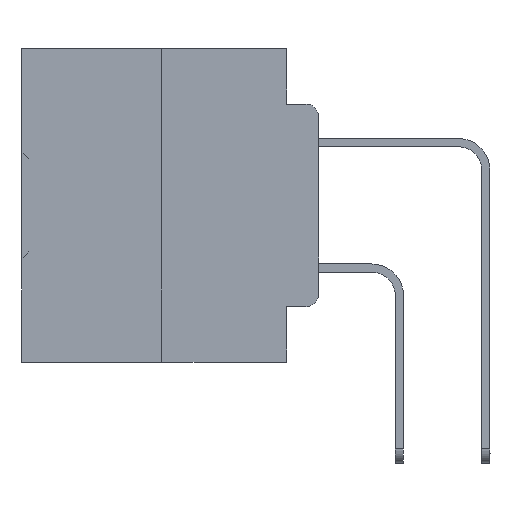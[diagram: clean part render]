
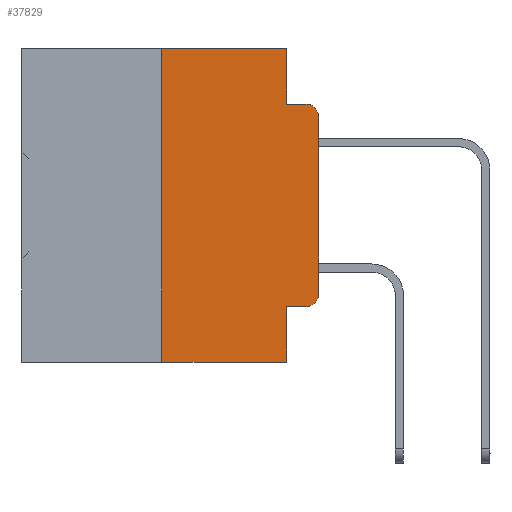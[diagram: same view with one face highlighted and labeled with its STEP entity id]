
A CAD part, left-side view. The second image highlights one B-rep face of the part: STEP entity #37829.
In plain terms, the highlighted planar face has unit normal (-1, 0, 0).
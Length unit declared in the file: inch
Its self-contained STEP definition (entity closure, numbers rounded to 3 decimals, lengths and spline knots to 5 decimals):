
#450 = ORIENTED_EDGE ( 'NONE', *, *, #13954, .F. ) ;
#592 = DIRECTION ( 'NONE',  ( 0., 0., 1. ) ) ;
#2484 = VECTOR ( 'NONE', #10250, 39.37008 ) ;
#3014 = DIRECTION ( 'NONE',  ( 1., 0., 0. ) ) ;
#3272 = VERTEX_POINT ( 'NONE', #13141 ) ;
#3385 = ORIENTED_EDGE ( 'NONE', *, *, #21034, .T. ) ;
#3446 = LINE ( 'NONE', #28257, #2484 ) ;
#3587 = EDGE_CURVE ( 'NONE', #24269, #38353, #11432, .T. ) ;
#4390 = ORIENTED_EDGE ( 'NONE', *, *, #3587, .T. ) ;
#4460 = DIRECTION ( 'NONE',  ( -1., 0., 0. ) ) ;
#5058 = CARTESIAN_POINT ( 'NONE',  ( 0., 0.051, -0.0885 ) ) ;
#5810 = ORIENTED_EDGE ( 'NONE', *, *, #15964, .F. ) ;
#6572 = CARTESIAN_POINT ( 'NONE',  ( 0., 0.25, 0. ) ) ;
#6968 = CARTESIAN_POINT ( 'NONE',  ( 0., 0., -0.3915 ) ) ;
#7860 = VERTEX_POINT ( 'NONE', #6968 ) ;
#8495 = CIRCLE ( 'NONE', #21261, 0.02 ) ;
#9760 = CARTESIAN_POINT ( 'NONE',  ( 0., 0.051, -0.0885 ) ) ;
#10250 = DIRECTION ( 'NONE',  ( 0., 0., 1. ) ) ;
#11415 = LINE ( 'NONE', #25062, #13327 ) ;
#11432 = LINE ( 'NONE', #21332, #25587 ) ;
#11882 = EDGE_CURVE ( 'NONE', #24269, #38934, #12449, .T. ) ;
#12086 = ORIENTED_EDGE ( 'NONE', *, *, #26048, .F. ) ;
#12449 = LINE ( 'NONE', #36280, #20502 ) ;
#12929 = DIRECTION ( 'NONE',  ( 0., -1., 0. ) ) ;
#13141 = CARTESIAN_POINT ( 'NONE',  ( 0., 0.25, -0.5 ) ) ;
#13247 = VECTOR ( 'NONE', #21427, 39.37008 ) ;
#13327 = VECTOR ( 'NONE', #592, 39.37008 ) ;
#13954 = EDGE_CURVE ( 'NONE', #3272, #18028, #11415, .T. ) ;
#15113 = VERTEX_POINT ( 'NONE', #5058 ) ;
#15505 = FACE_OUTER_BOUND ( 'NONE', #34352, .T. ) ;
#15509 = CARTESIAN_POINT ( 'NONE',  ( 0., 0.473, 0. ) ) ;
#15949 = LINE ( 'NONE', #22445, #30944 ) ;
#15964 = EDGE_CURVE ( 'NONE', #21119, #15113, #28658, .T. ) ;
#16510 = CARTESIAN_POINT ( 'NONE',  ( 0., 0., -0.1085 ) ) ;
#17420 = PLANE ( 'NONE',  #22831 ) ;
#17607 = CARTESIAN_POINT ( 'NONE',  ( 0., 0.02, -0.0885 ) ) ;
#17874 = LINE ( 'NONE', #9760, #24015 ) ;
#18028 = VERTEX_POINT ( 'NONE', #6572 ) ;
#18172 = CARTESIAN_POINT ( 'NONE',  ( 0., 0.02, -0.1085 ) ) ;
#18179 = VERTEX_POINT ( 'NONE', #16510 ) ;
#18267 = DIRECTION ( 'NONE',  ( 0., -1., 0. ) ) ;
#19278 = EDGE_CURVE ( 'NONE', #18028, #21119, #29210, .T. ) ;
#19913 = CARTESIAN_POINT ( 'NONE',  ( 0., 0.051, -0.4115 ) ) ;
#20502 = VECTOR ( 'NONE', #39207, 39.37008 ) ;
#20570 = AXIS2_PLACEMENT_3D ( 'NONE', #22721, #4460, #25741 ) ;
#20704 = VECTOR ( 'NONE', #27346, 39.37008 ) ;
#21034 = EDGE_CURVE ( 'NONE', #3272, #38934, #15949, .T. ) ;
#21119 = VERTEX_POINT ( 'NONE', #31861 ) ;
#21241 = DIRECTION ( 'NONE',  ( 0., 0., -1. ) ) ;
#21261 = AXIS2_PLACEMENT_3D ( 'NONE', #18172, #39087, #21241 ) ;
#21332 = CARTESIAN_POINT ( 'NONE',  ( 0., 0.051, -0.4115 ) ) ;
#21427 = DIRECTION ( 'NONE',  ( 0., -1., 0. ) ) ;
#21566 = ORIENTED_EDGE ( 'NONE', *, *, #38753, .T. ) ;
#22025 = ORIENTED_EDGE ( 'NONE', *, *, #19278, .F. ) ;
#22445 = CARTESIAN_POINT ( 'NONE',  ( 0., 0.473, -0.5 ) ) ;
#22721 = CARTESIAN_POINT ( 'NONE',  ( 0., 0.02, -0.3915 ) ) ;
#22831 = AXIS2_PLACEMENT_3D ( 'NONE', #23510, #3014, #24365 ) ;
#23510 = CARTESIAN_POINT ( 'NONE',  ( 0., 0.473, 0. ) ) ;
#24015 = VECTOR ( 'NONE', #12929, 39.37008 ) ;
#24269 = VERTEX_POINT ( 'NONE', #19913 ) ;
#24365 = DIRECTION ( 'NONE',  ( 0., 0., -1. ) ) ;
#24397 = CARTESIAN_POINT ( 'NONE',  ( 0., 0.051, 0. ) ) ;
#25062 = CARTESIAN_POINT ( 'NONE',  ( 0., 0.25, 0. ) ) ;
#25323 = ORIENTED_EDGE ( 'NONE', *, *, #38032, .T. ) ;
#25487 = DIRECTION ( 'NONE',  ( 0., -1., 0. ) ) ;
#25587 = VECTOR ( 'NONE', #18267, 39.37008 ) ;
#25741 = DIRECTION ( 'NONE',  ( 0., 0., -1. ) ) ;
#26048 = EDGE_CURVE ( 'NONE', #15113, #34246, #17874, .T. ) ;
#27140 = ORIENTED_EDGE ( 'NONE', *, *, #36038, .T. ) ;
#27346 = DIRECTION ( 'NONE',  ( 0., 0., -1. ) ) ;
#28257 = CARTESIAN_POINT ( 'NONE',  ( 0., 0., 0. ) ) ;
#28658 = LINE ( 'NONE', #24397, #20704 ) ;
#29210 = LINE ( 'NONE', #15509, #13247 ) ;
#29623 = CARTESIAN_POINT ( 'NONE',  ( 0., 0.051, -0.5 ) ) ;
#30433 = CIRCLE ( 'NONE', #20570, 0.02 ) ;
#30944 = VECTOR ( 'NONE', #25487, 39.37008 ) ;
#31861 = CARTESIAN_POINT ( 'NONE',  ( 0., 0.051, 0. ) ) ;
#34246 = VERTEX_POINT ( 'NONE', #17607 ) ;
#34352 = EDGE_LOOP ( 'NONE', ( #25323, #27140, #12086, #5810, #22025, #450, #3385, #35620, #4390, #21566 ) ) ;
#35567 = CARTESIAN_POINT ( 'NONE',  ( 0., 0.02, -0.4115 ) ) ;
#35620 = ORIENTED_EDGE ( 'NONE', *, *, #11882, .F. ) ;
#36038 = EDGE_CURVE ( 'NONE', #18179, #34246, #8495, .T. ) ;
#36280 = CARTESIAN_POINT ( 'NONE',  ( 0., 0.051, 0. ) ) ;
#37829 = ADVANCED_FACE ( 'NONE', ( #15505 ), #17420, .F. ) ;
#38032 = EDGE_CURVE ( 'NONE', #7860, #18179, #3446, .T. ) ;
#38353 = VERTEX_POINT ( 'NONE', #35567 ) ;
#38753 = EDGE_CURVE ( 'NONE', #38353, #7860, #30433, .T. ) ;
#38934 = VERTEX_POINT ( 'NONE', #29623 ) ;
#39087 = DIRECTION ( 'NONE',  ( -1., 0., 0. ) ) ;
#39207 = DIRECTION ( 'NONE',  ( 0., 0., -1. ) ) ;
